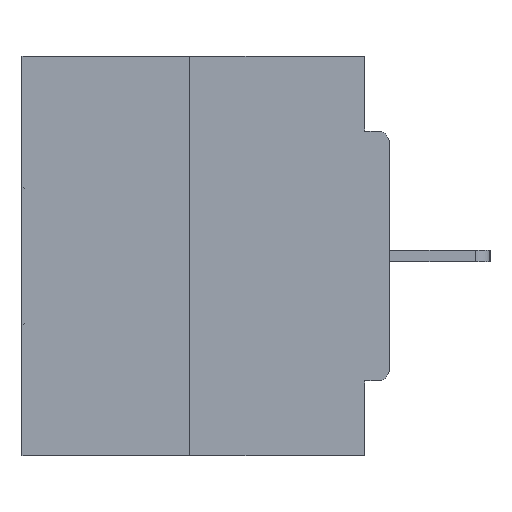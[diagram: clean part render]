
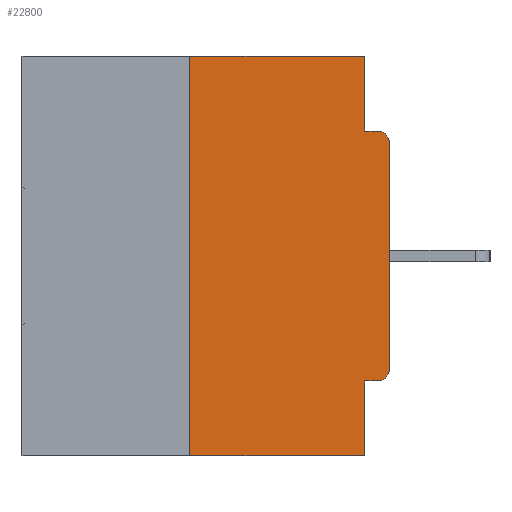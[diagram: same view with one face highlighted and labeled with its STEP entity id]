
A CAD part, left-side view. The second image highlights one B-rep face of the part: STEP entity #22800.
In plain terms, the highlighted planar face has unit normal (-1, 0, 0).
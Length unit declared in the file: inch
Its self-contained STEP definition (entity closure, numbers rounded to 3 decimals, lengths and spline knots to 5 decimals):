
#897 = DIRECTION ( 'NONE',  ( 0., -1., 0. ) ) ;
#962 = VERTEX_POINT ( 'NONE', #30140 ) ;
#1582 = CIRCLE ( 'NONE', #17438, 0.015 ) ;
#1603 = PLANE ( 'NONE',  #29732 ) ;
#1663 = CARTESIAN_POINT ( 'NONE',  ( 0., 0.031, 0. ) ) ;
#1886 = DIRECTION ( 'NONE',  ( -1., 0., 0. ) ) ;
#1893 = VERTEX_POINT ( 'NONE', #11240 ) ;
#2229 = ORIENTED_EDGE ( 'NONE', *, *, #20515, .F. ) ;
#3508 = DIRECTION ( 'NONE',  ( 0., 0., 1. ) ) ;
#3589 = EDGE_CURVE ( 'NONE', #12812, #1893, #9546, .T. ) ;
#3791 = EDGE_LOOP ( 'NONE', ( #28899, #2229, #3822, #20605, #33793, #33048, #11260, #25743, #29184, #27199 ) ) ;
#3822 = ORIENTED_EDGE ( 'NONE', *, *, #28454, .T. ) ;
#6090 = EDGE_CURVE ( 'NONE', #14047, #21008, #17402, .T. ) ;
#6369 = EDGE_CURVE ( 'NONE', #34641, #12812, #26100, .T. ) ;
#6649 = VECTOR ( 'NONE', #28059, 39.37008 ) ;
#6673 = DIRECTION ( 'NONE',  ( 0., 0., -1. ) ) ;
#6969 = CARTESIAN_POINT ( 'NONE',  ( 0., 0.031, -0.5 ) ) ;
#7371 = VECTOR ( 'NONE', #15421, 39.37008 ) ;
#7592 = DIRECTION ( 'NONE',  ( 0., 0., -1. ) ) ;
#8211 = CARTESIAN_POINT ( 'NONE',  ( 0., 0., 0. ) ) ;
#8297 = CARTESIAN_POINT ( 'NONE',  ( 0., 0., -0.0935 ) ) ;
#9030 = VERTEX_POINT ( 'NONE', #24798 ) ;
#9083 = DIRECTION ( 'NONE',  ( 0., 1., 0. ) ) ;
#9546 = LINE ( 'NONE', #1663, #26812 ) ;
#10174 = CARTESIAN_POINT ( 'NONE',  ( 0., 0., -0.3915 ) ) ;
#10956 = DIRECTION ( 'NONE',  ( 0., -1., 0. ) ) ;
#11240 = CARTESIAN_POINT ( 'NONE',  ( 0., 0.031, -0.0935 ) ) ;
#11260 = ORIENTED_EDGE ( 'NONE', *, *, #30169, .T. ) ;
#12510 = CARTESIAN_POINT ( 'NONE',  ( 0., 0.015, -0.1085 ) ) ;
#12523 = VERTEX_POINT ( 'NONE', #10174 ) ;
#12812 = VERTEX_POINT ( 'NONE', #34382 ) ;
#13801 = CARTESIAN_POINT ( 'NONE',  ( 0., 0.46, 0. ) ) ;
#14047 = VERTEX_POINT ( 'NONE', #18243 ) ;
#14823 = CARTESIAN_POINT ( 'NONE',  ( 0., 0.015, -0.0935 ) ) ;
#15421 = DIRECTION ( 'NONE',  ( 0., 0., -1. ) ) ;
#16249 = AXIS2_PLACEMENT_3D ( 'NONE', #12510, #34387, #6673 ) ;
#17227 = VECTOR ( 'NONE', #10956, 39.37008 ) ;
#17402 = CIRCLE ( 'NONE', #16249, 0.015 ) ;
#17438 = AXIS2_PLACEMENT_3D ( 'NONE', #19358, #1886, #7592 ) ;
#17635 = LINE ( 'NONE', #6969, #7371 ) ;
#17784 = CARTESIAN_POINT ( 'NONE',  ( 0., 0.46, 0. ) ) ;
#17939 = EDGE_CURVE ( 'NONE', #9030, #19059, #23085, .T. ) ;
#17963 = DIRECTION ( 'NONE',  ( 1., 0., 0. ) ) ;
#18243 = CARTESIAN_POINT ( 'NONE',  ( 0., 0., -0.1085 ) ) ;
#18502 = FACE_OUTER_BOUND ( 'NONE', #3791, .T. ) ;
#19059 = VERTEX_POINT ( 'NONE', #30821 ) ;
#19358 = CARTESIAN_POINT ( 'NONE',  ( 0., 0.015, -0.3915 ) ) ;
#19360 = DIRECTION ( 'NONE',  ( 0., -1., 0. ) ) ;
#20515 = EDGE_CURVE ( 'NONE', #962, #34641, #31636, .T. ) ;
#20605 = ORIENTED_EDGE ( 'NONE', *, *, #23407, .F. ) ;
#21008 = VERTEX_POINT ( 'NONE', #14823 ) ;
#21137 = DIRECTION ( 'NONE',  ( 0., 0., -1. ) ) ;
#22800 = ADVANCED_FACE ( 'NONE', ( #18502 ), #1603, .F. ) ;
#23085 = LINE ( 'NONE', #25671, #30024 ) ;
#23407 = EDGE_CURVE ( 'NONE', #19059, #33393, #17635, .T. ) ;
#24798 = CARTESIAN_POINT ( 'NONE',  ( 0., 0.015, -0.4065 ) ) ;
#25671 = CARTESIAN_POINT ( 'NONE',  ( 0., 0., -0.4065 ) ) ;
#25743 = ORIENTED_EDGE ( 'NONE', *, *, #6090, .T. ) ;
#26100 = LINE ( 'NONE', #13801, #28279 ) ;
#26812 = VECTOR ( 'NONE', #21137, 39.37008 ) ;
#27199 = ORIENTED_EDGE ( 'NONE', *, *, #3589, .F. ) ;
#27269 = VECTOR ( 'NONE', #3508, 39.37008 ) ;
#28059 = DIRECTION ( 'NONE',  ( 0., 0., 1. ) ) ;
#28095 = LINE ( 'NONE', #36152, #17227 ) ;
#28279 = VECTOR ( 'NONE', #897, 39.37008 ) ;
#28454 = EDGE_CURVE ( 'NONE', #962, #33393, #28095, .T. ) ;
#28523 = CARTESIAN_POINT ( 'NONE',  ( 0., 0.031, -0.5 ) ) ;
#28899 = ORIENTED_EDGE ( 'NONE', *, *, #6369, .F. ) ;
#28977 = DIRECTION ( 'NONE',  ( 0., 0., -1. ) ) ;
#29184 = ORIENTED_EDGE ( 'NONE', *, *, #31011, .F. ) ;
#29732 = AXIS2_PLACEMENT_3D ( 'NONE', #17784, #17963, #28977 ) ;
#30024 = VECTOR ( 'NONE', #9083, 39.37008 ) ;
#30140 = CARTESIAN_POINT ( 'NONE',  ( 0., 0.25, -0.5 ) ) ;
#30169 = EDGE_CURVE ( 'NONE', #12523, #14047, #33362, .T. ) ;
#30821 = CARTESIAN_POINT ( 'NONE',  ( 0., 0.031, -0.4065 ) ) ;
#31011 = EDGE_CURVE ( 'NONE', #1893, #21008, #33448, .T. ) ;
#31636 = LINE ( 'NONE', #34360, #27269 ) ;
#31929 = VECTOR ( 'NONE', #19360, 39.37008 ) ;
#33048 = ORIENTED_EDGE ( 'NONE', *, *, #33757, .T. ) ;
#33362 = LINE ( 'NONE', #8211, #6649 ) ;
#33374 = CARTESIAN_POINT ( 'NONE',  ( 0., 0.25, 0. ) ) ;
#33393 = VERTEX_POINT ( 'NONE', #28523 ) ;
#33448 = LINE ( 'NONE', #8297, #31929 ) ;
#33757 = EDGE_CURVE ( 'NONE', #9030, #12523, #1582, .T. ) ;
#33793 = ORIENTED_EDGE ( 'NONE', *, *, #17939, .F. ) ;
#34360 = CARTESIAN_POINT ( 'NONE',  ( 0., 0.25, 0. ) ) ;
#34382 = CARTESIAN_POINT ( 'NONE',  ( 0., 0.031, 0. ) ) ;
#34387 = DIRECTION ( 'NONE',  ( -1., 0., 0. ) ) ;
#34641 = VERTEX_POINT ( 'NONE', #33374 ) ;
#36152 = CARTESIAN_POINT ( 'NONE',  ( 0., 0.46, -0.5 ) ) ;
